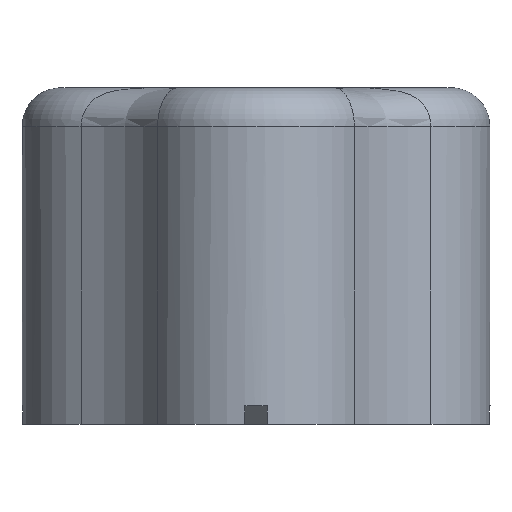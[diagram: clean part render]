
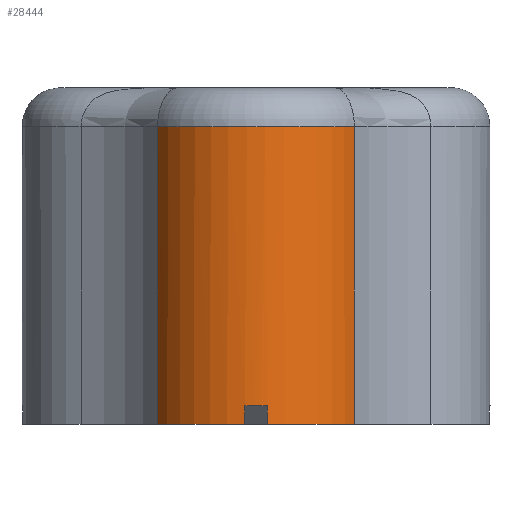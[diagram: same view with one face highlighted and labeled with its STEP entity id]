
A CAD part, left-side view. The second image highlights one B-rep face of the part: STEP entity #28444.
In plain terms, the highlighted cylindrical face has radius 15 mm (diameter 30 mm), a partial arc.
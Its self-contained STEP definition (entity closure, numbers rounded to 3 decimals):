
#309 = CARTESIAN_POINT ( 'NONE',  ( -31.391, -14.966, 2.462 ) ) ;
#1410 = VERTEX_POINT ( 'NONE', #9718 ) ;
#2228 = VERTEX_POINT ( 'NONE', #35967 ) ;
#2932 = CARTESIAN_POINT ( 'NONE',  ( -31.391, -14.966, 2.462 ) ) ;
#3661 = DIRECTION ( 'NONE',  ( 0., 0., -1. ) ) ;
#4024 = ORIENTED_EDGE ( 'NONE', *, *, #54366, .T. ) ;
#4953 = EDGE_CURVE ( 'NONE', #61603, #13621, #11952, .T. ) ;
#5223 = CARTESIAN_POINT ( 'NONE',  ( -31.391, -17.966, 40. ) ) ;
#6808 = CYLINDRICAL_SURFACE ( 'NONE', #42182, 15. ) ;
#9718 = CARTESIAN_POINT ( 'NONE',  ( -23.526, -3.232, 0. ) ) ;
#11559 = VECTOR ( 'NONE', #66513, 1000. ) ;
#11952 =( BOUNDED_CURVE ( )  B_SPLINE_CURVE ( 3, ( #2932, #68831, #57797, #41441 ),
 .UNSPECIFIED., .F., .F. ) 
 B_SPLINE_CURVE_WITH_KNOTS ( ( 4, 4 ),
 ( 3.041, 3.242 ),
 .UNSPECIFIED. ) 
 CURVE ( )  GEOMETRIC_REPRESENTATION_ITEM ( )  RATIONAL_B_SPLINE_CURVE ( ( 1., 0.997, 0.997, 1. ) ) 
 REPRESENTATION_ITEM ( '' )  );
#12123 = CARTESIAN_POINT ( 'NONE',  ( -23.526, -29.701, 0. ) ) ;
#13440 = ORIENTED_EDGE ( 'NONE', *, *, #13771, .T. ) ;
#13621 = VERTEX_POINT ( 'NONE', #22636 ) ;
#13771 = EDGE_CURVE ( 'NONE', #13621, #49022, #40774, .T. ) ;
#14711 = ORIENTED_EDGE ( 'NONE', *, *, #52208, .T. ) ;
#15037 = CIRCLE ( 'NONE', #47554, 15. ) ;
#15661 = LINE ( 'NONE', #58544, #59551 ) ;
#15864 = AXIS2_PLACEMENT_3D ( 'NONE', #30223, #68731, #35765 ) ;
#17128 = CARTESIAN_POINT ( 'NONE',  ( -23.526, -29.701, 40. ) ) ;
#17347 = CARTESIAN_POINT ( 'NONE',  ( -16.466, -16.466, 0. ) ) ;
#17576 = ORIENTED_EDGE ( 'NONE', *, *, #66524, .T. ) ;
#19263 = CIRCLE ( 'NONE', #21723, 15. ) ;
#21723 = AXIS2_PLACEMENT_3D ( 'NONE', #64434, #31466, #69961 ) ;
#22636 = CARTESIAN_POINT ( 'NONE',  ( -31.391, -17.966, 2.462 ) ) ;
#22860 = DIRECTION ( 'NONE',  ( 0., 1., 0. ) ) ;
#24203 = CARTESIAN_POINT ( 'NONE',  ( -23.526, -29.701, 40. ) ) ;
#27793 = LINE ( 'NONE', #64935, #55357 ) ;
#28444 = ADVANCED_FACE ( 'NONE', ( #37781 ), #6808, .T. ) ;
#29923 = LINE ( 'NONE', #24203, #57508 ) ;
#29982 = EDGE_CURVE ( 'NONE', #52865, #40261, #29923, .T. ) ;
#30223 = CARTESIAN_POINT ( 'NONE',  ( -16.466, -16.466, 0. ) ) ;
#31466 = DIRECTION ( 'NONE',  ( 0., 0., -1. ) ) ;
#32483 = EDGE_CURVE ( 'NONE', #2228, #1410, #15661, .T. ) ;
#33025 = DIRECTION ( 'NONE',  ( 0., -1., 0. ) ) ;
#33046 = ORIENTED_EDGE ( 'NONE', *, *, #29982, .T. ) ;
#34175 = CARTESIAN_POINT ( 'NONE',  ( -31.391, -14.966, 0. ) ) ;
#35765 = DIRECTION ( 'NONE',  ( 0., 1., 0. ) ) ;
#35967 = CARTESIAN_POINT ( 'NONE',  ( -23.526, -3.232, 40. ) ) ;
#37781 = FACE_OUTER_BOUND ( 'NONE', #59011, .T. ) ;
#40261 = VERTEX_POINT ( 'NONE', #17128 ) ;
#40774 = LINE ( 'NONE', #5223, #11559 ) ;
#41441 = CARTESIAN_POINT ( 'NONE',  ( -31.391, -17.966, 2.462 ) ) ;
#42182 = AXIS2_PLACEMENT_3D ( 'NONE', #49440, #44112, #33025 ) ;
#44112 = DIRECTION ( 'NONE',  ( 0., 0., -1. ) ) ;
#45336 = ORIENTED_EDGE ( 'NONE', *, *, #32483, .T. ) ;
#45666 = CARTESIAN_POINT ( 'NONE',  ( -31.391, -17.966, 0. ) ) ;
#47554 = AXIS2_PLACEMENT_3D ( 'NONE', #17347, #55865, #22860 ) ;
#48074 = ORIENTED_EDGE ( 'NONE', *, *, #63321, .T. ) ;
#49022 = VERTEX_POINT ( 'NONE', #45666 ) ;
#49440 = CARTESIAN_POINT ( 'NONE',  ( -16.466, -16.466, 40. ) ) ;
#51398 = DIRECTION ( 'NONE',  ( 0., 0., 1. ) ) ;
#52050 = VERTEX_POINT ( 'NONE', #34175 ) ;
#52208 = EDGE_CURVE ( 'NONE', #40261, #2228, #19263, .T. ) ;
#52865 = VERTEX_POINT ( 'NONE', #12123 ) ;
#54366 = EDGE_CURVE ( 'NONE', #1410, #52050, #69092, .T. ) ;
#55357 = VECTOR ( 'NONE', #70480, 1000. ) ;
#55865 = DIRECTION ( 'NONE',  ( 0., 0., 1. ) ) ;
#57508 = VECTOR ( 'NONE', #51398, 1000. ) ;
#57797 = CARTESIAN_POINT ( 'NONE',  ( -31.492, -16.968, 2.513 ) ) ;
#58544 = CARTESIAN_POINT ( 'NONE',  ( -23.526, -3.232, 40. ) ) ;
#59011 = EDGE_LOOP ( 'NONE', ( #4024, #17576, #66132, #13440, #48074, #33046, #14711, #45336 ) ) ;
#59551 = VECTOR ( 'NONE', #3661, 1000. ) ;
#61603 = VERTEX_POINT ( 'NONE', #309 ) ;
#63321 = EDGE_CURVE ( 'NONE', #49022, #52865, #15037, .T. ) ;
#64434 = CARTESIAN_POINT ( 'NONE',  ( -16.466, -16.466, 40. ) ) ;
#64935 = CARTESIAN_POINT ( 'NONE',  ( -31.391, -14.966, 40. ) ) ;
#66132 = ORIENTED_EDGE ( 'NONE', *, *, #4953, .T. ) ;
#66513 = DIRECTION ( 'NONE',  ( 0., 0., -1. ) ) ;
#66524 = EDGE_CURVE ( 'NONE', #52050, #61603, #27793, .T. ) ;
#68731 = DIRECTION ( 'NONE',  ( 0., 0., 1. ) ) ;
#68831 = CARTESIAN_POINT ( 'NONE',  ( -31.492, -15.965, 2.513 ) ) ;
#69092 = CIRCLE ( 'NONE', #15864, 15. ) ;
#69961 = DIRECTION ( 'NONE',  ( 0., 1., 0. ) ) ;
#70480 = DIRECTION ( 'NONE',  ( 0., 0., 1. ) ) ;
